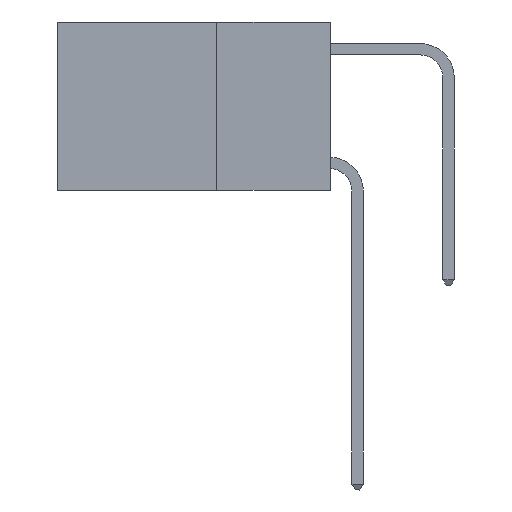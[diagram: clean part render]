
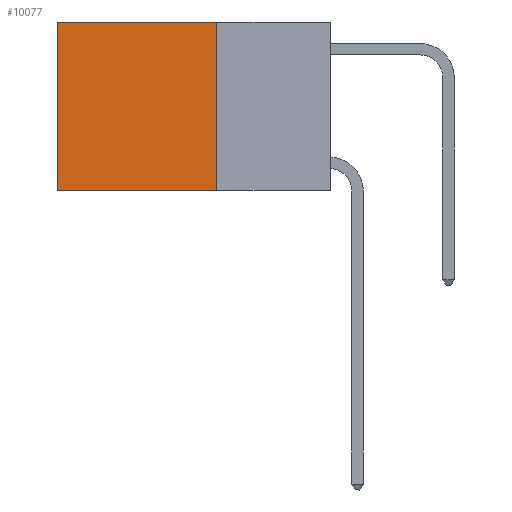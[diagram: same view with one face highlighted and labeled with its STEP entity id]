
A CAD part, left-side view. The second image highlights one B-rep face of the part: STEP entity #10077.
In plain terms, the highlighted planar face has unit normal (-1, 0, 0).
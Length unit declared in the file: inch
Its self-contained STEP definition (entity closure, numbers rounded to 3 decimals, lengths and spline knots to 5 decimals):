
#179 = DIRECTION ( 'NONE',  ( 0., 1., 0. ) ) ;
#834 = CARTESIAN_POINT ( 'NONE',  ( 0.2625, 0.6, 0. ) ) ;
#1614 = DIRECTION ( 'NONE',  ( 1., 0., 0. ) ) ;
#1699 = LINE ( 'NONE', #6150, #10096 ) ;
#2023 = VERTEX_POINT ( 'NONE', #834 ) ;
#2899 = PLANE ( 'NONE',  #11680 ) ;
#3594 = VECTOR ( 'NONE', #179, 39.37008 ) ;
#4617 = LINE ( 'NONE', #13691, #3594 ) ;
#4828 = LINE ( 'NONE', #11460, #11031 ) ;
#5142 = VERTEX_POINT ( 'NONE', #11541 ) ;
#5254 = CARTESIAN_POINT ( 'NONE',  ( 0.2625, 0.6, 0. ) ) ;
#5638 = EDGE_LOOP ( 'NONE', ( #5833, #5786, #10823, #12447 ) ) ;
#5786 = ORIENTED_EDGE ( 'NONE', *, *, #12869, .F. ) ;
#5833 = ORIENTED_EDGE ( 'NONE', *, *, #6567, .T. ) ;
#6150 = CARTESIAN_POINT ( 'NONE',  ( 0.2625, 0.25, -0.37 ) ) ;
#6354 = VERTEX_POINT ( 'NONE', #11126 ) ;
#6567 = EDGE_CURVE ( 'NONE', #2023, #10727, #9560, .T. ) ;
#8166 = EDGE_CURVE ( 'NONE', #5142, #2023, #4617, .T. ) ;
#9553 = FACE_OUTER_BOUND ( 'NONE', #5638, .T. ) ;
#9560 = LINE ( 'NONE', #5254, #14256 ) ;
#9640 = DIRECTION ( 'NONE',  ( 0., 1., 0. ) ) ;
#9707 = DIRECTION ( 'NONE',  ( 0., 0., -1. ) ) ;
#10077 = ADVANCED_FACE ( 'NONE', ( #9553 ), #2899, .F. ) ;
#10096 = VECTOR ( 'NONE', #9640, 39.37008 ) ;
#10293 = DIRECTION ( 'NONE',  ( 0., 0., -1. ) ) ;
#10727 = VERTEX_POINT ( 'NONE', #10942 ) ;
#10823 = ORIENTED_EDGE ( 'NONE', *, *, #12331, .F. ) ;
#10942 = CARTESIAN_POINT ( 'NONE',  ( 0.2625, 0.6, -0.37 ) ) ;
#11031 = VECTOR ( 'NONE', #10293, 39.37008 ) ;
#11126 = CARTESIAN_POINT ( 'NONE',  ( 0.2625, 0.25, -0.37 ) ) ;
#11460 = CARTESIAN_POINT ( 'NONE',  ( 0.2625, 0.25, 0. ) ) ;
#11541 = CARTESIAN_POINT ( 'NONE',  ( 0.2625, 0.25, 0. ) ) ;
#11680 = AXIS2_PLACEMENT_3D ( 'NONE', #14083, #1614, #9707 ) ;
#11797 = DIRECTION ( 'NONE',  ( 0., 0., -1. ) ) ;
#12331 = EDGE_CURVE ( 'NONE', #5142, #6354, #4828, .T. ) ;
#12447 = ORIENTED_EDGE ( 'NONE', *, *, #8166, .T. ) ;
#12869 = EDGE_CURVE ( 'NONE', #6354, #10727, #1699, .T. ) ;
#13691 = CARTESIAN_POINT ( 'NONE',  ( 0.2625, 0.25, 0. ) ) ;
#14083 = CARTESIAN_POINT ( 'NONE',  ( 0.2625, 0.25, 0. ) ) ;
#14256 = VECTOR ( 'NONE', #11797, 39.37008 ) ;
